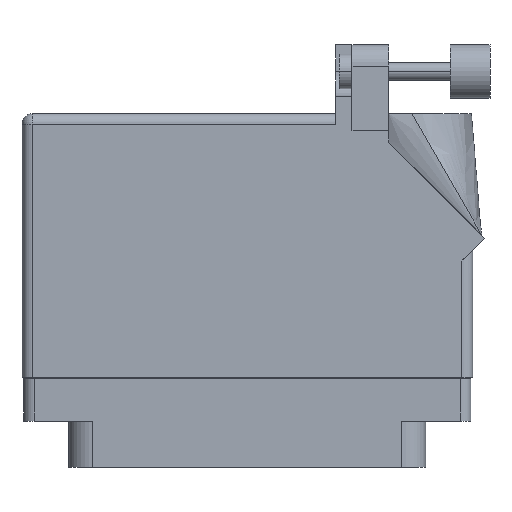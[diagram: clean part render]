
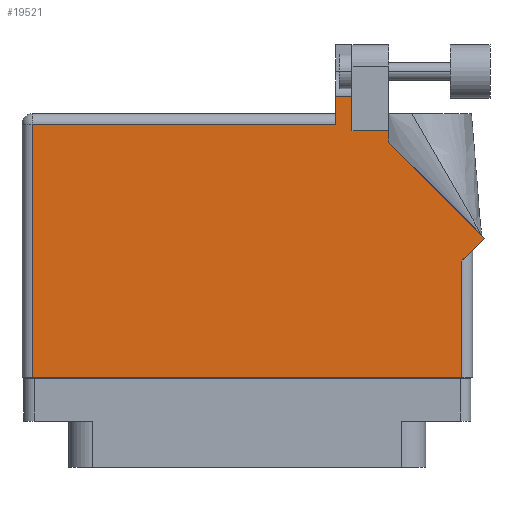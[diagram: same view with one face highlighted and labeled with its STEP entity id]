
A CAD part, front view. The second image highlights one B-rep face of the part: STEP entity #19521.
In plain terms, the highlighted face is planar.
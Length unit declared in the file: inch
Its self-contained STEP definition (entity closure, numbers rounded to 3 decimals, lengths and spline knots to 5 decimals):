
#1962 = DIRECTION ( 'NONE',  ( 0., 1., 0. ) ) ;
#2339 = EDGE_CURVE ( 'NONE', #6748, #19665, #34477, .T. ) ;
#2669 = CARTESIAN_POINT ( 'NONE',  ( -1.306, 1.43, 0.455 ) ) ;
#3012 = PLANE ( 'NONE',  #7684 ) ;
#3174 = ORIENTED_EDGE ( 'NONE', *, *, #38565, .T. ) ;
#3584 = VECTOR ( 'NONE', #25894, 39.37008 ) ;
#3773 = EDGE_CURVE ( 'NONE', #25743, #36689, #9255, .T. ) ;
#3929 = LINE ( 'NONE', #26115, #22565 ) ;
#4601 = CARTESIAN_POINT ( 'NONE',  ( 1.306, 0.637, 0.455 ) ) ;
#5706 = VERTEX_POINT ( 'NONE', #46223 ) ;
#6131 = VECTOR ( 'NONE', #9274, 39.37008 ) ;
#6232 = VECTOR ( 'NONE', #1962, 39.37008 ) ;
#6748 = VERTEX_POINT ( 'NONE', #35886 ) ;
#7314 = ORIENTED_EDGE ( 'NONE', *, *, #37489, .T. ) ;
#7577 = EDGE_LOOP ( 'NONE', ( #7810, #12627, #3174, #16935, #26036, #46610, #27116, #7314, #31782, #34370, #25697 ) ) ;
#7684 = AXIS2_PLACEMENT_3D ( 'NONE', #2669, #29329, #25422 ) ;
#7810 = ORIENTED_EDGE ( 'NONE', *, *, #2339, .T. ) ;
#8013 = DIRECTION ( 'NONE',  ( 1., 0., 0. ) ) ;
#8032 = CARTESIAN_POINT ( 'NONE',  ( 1.244, -0.1, 0.455 ) ) ;
#8064 = VECTOR ( 'NONE', #38087, 39.37008 ) ;
#8741 = VECTOR ( 'NONE', #31526, 39.37008 ) ;
#8875 = VERTEX_POINT ( 'NONE', #41855 ) ;
#9255 = LINE ( 'NONE', #45515, #46002 ) ;
#9274 = DIRECTION ( 'NONE',  ( 0., -1., 0. ) ) ;
#9594 = LINE ( 'NONE', #24406, #6131 ) ;
#9969 = CARTESIAN_POINT ( 'NONE',  ( 1.37671, 0.70771, 0.455 ) ) ;
#12627 = ORIENTED_EDGE ( 'NONE', *, *, #42605, .T. ) ;
#14655 = CARTESIAN_POINT ( 'NONE',  ( 0.93777, 1.5315, 0.455 ) ) ;
#16114 = DIRECTION ( 'NONE',  ( 0.707, 0.707, 0. ) ) ;
#16935 = ORIENTED_EDGE ( 'NONE', *, *, #20073, .T. ) ;
#17822 = EDGE_CURVE ( 'NONE', #8875, #25743, #9594, .T. ) ;
#17823 = VECTOR ( 'NONE', #35160, 39.37008 ) ;
#18857 = CARTESIAN_POINT ( 'NONE',  ( 0.607, 1.33, 0.455 ) ) ;
#19242 = VERTEX_POINT ( 'NONE', #34179 ) ;
#19521 = ADVANCED_FACE ( 'NONE', ( #28025 ), #3012, .F. ) ;
#19665 = VERTEX_POINT ( 'NONE', #40789 ) ;
#20073 = EDGE_CURVE ( 'NONE', #5706, #8875, #26042, .T. ) ;
#20743 = CARTESIAN_POINT ( 'NONE',  ( 0.513, 1.43, 0.455 ) ) ;
#20797 = EDGE_CURVE ( 'NONE', #36689, #28639, #38852, .T. ) ;
#22565 = VECTOR ( 'NONE', #33324, 39.37008 ) ;
#23106 = LINE ( 'NONE', #4601, #41181 ) ;
#23268 = CARTESIAN_POINT ( 'NONE',  ( -1.306, 1.368, 0.455 ) ) ;
#24132 = VERTEX_POINT ( 'NONE', #33546 ) ;
#24406 = CARTESIAN_POINT ( 'NONE',  ( -1.244, -0.1, 0.455 ) ) ;
#24574 = CARTESIAN_POINT ( 'NONE',  ( 1.244, 0.637, 0.455 ) ) ;
#24589 = CARTESIAN_POINT ( 'NONE',  ( 0.82, 1.33, 0.455 ) ) ;
#25422 = DIRECTION ( 'NONE',  ( -1., 0., 0. ) ) ;
#25697 = ORIENTED_EDGE ( 'NONE', *, *, #32283, .T. ) ;
#25743 = VERTEX_POINT ( 'NONE', #42292 ) ;
#25832 = DIRECTION ( 'NONE',  ( 0., 1., 0. ) ) ;
#25894 = DIRECTION ( 'NONE',  ( -1., 0., 0. ) ) ;
#26036 = ORIENTED_EDGE ( 'NONE', *, *, #17822, .T. ) ;
#26042 = LINE ( 'NONE', #23268, #8064 ) ;
#26115 = CARTESIAN_POINT ( 'NONE',  ( 0.82, 1.33, 0.455 ) ) ;
#27116 = ORIENTED_EDGE ( 'NONE', *, *, #20797, .T. ) ;
#27328 = VERTEX_POINT ( 'NONE', #46500 ) ;
#28025 = FACE_OUTER_BOUND ( 'NONE', #7577, .T. ) ;
#28639 = VERTEX_POINT ( 'NONE', #45467 ) ;
#29329 = DIRECTION ( 'NONE',  ( 0., 0., -1. ) ) ;
#29850 = VERTEX_POINT ( 'NONE', #24589 ) ;
#31526 = DIRECTION ( 'NONE',  ( 0., -1., 0. ) ) ;
#31782 = ORIENTED_EDGE ( 'NONE', *, *, #35930, .T. ) ;
#32128 = VECTOR ( 'NONE', #25832, 39.37008 ) ;
#32283 = EDGE_CURVE ( 'NONE', #29850, #6748, #3929, .T. ) ;
#32294 = DIRECTION ( 'NONE',  ( -0.707, 0.707, 0. ) ) ;
#32341 = LINE ( 'NONE', #20743, #8741 ) ;
#33324 = DIRECTION ( 'NONE',  ( -1., 0., 0. ) ) ;
#33546 = CARTESIAN_POINT ( 'NONE',  ( 1.37671, 0.70771, 0.455 ) ) ;
#34070 = EDGE_CURVE ( 'NONE', #19242, #29850, #44072, .T. ) ;
#34179 = CARTESIAN_POINT ( 'NONE',  ( 0.82, 1.26442, 0.455 ) ) ;
#34370 = ORIENTED_EDGE ( 'NONE', *, *, #34070, .T. ) ;
#34477 = LINE ( 'NONE', #18857, #32128 ) ;
#35160 = DIRECTION ( 'NONE',  ( 0., 1., 0. ) ) ;
#35848 = VECTOR ( 'NONE', #32294, 39.37008 ) ;
#35886 = CARTESIAN_POINT ( 'NONE',  ( 0.607, 1.33, 0.455 ) ) ;
#35930 = EDGE_CURVE ( 'NONE', #24132, #19242, #39918, .T. ) ;
#36689 = VERTEX_POINT ( 'NONE', #8032 ) ;
#36805 = LINE ( 'NONE', #14655, #3584 ) ;
#37489 = EDGE_CURVE ( 'NONE', #28639, #24132, #23106, .T. ) ;
#38087 = DIRECTION ( 'NONE',  ( -1., 0., 0. ) ) ;
#38565 = EDGE_CURVE ( 'NONE', #27328, #5706, #32341, .T. ) ;
#38852 = LINE ( 'NONE', #24574, #6232 ) ;
#39918 = LINE ( 'NONE', #9969, #35848 ) ;
#40789 = CARTESIAN_POINT ( 'NONE',  ( 0.607, 1.5315, 0.455 ) ) ;
#41181 = VECTOR ( 'NONE', #16114, 39.37008 ) ;
#41855 = CARTESIAN_POINT ( 'NONE',  ( -1.244, 1.368, 0.455 ) ) ;
#42292 = CARTESIAN_POINT ( 'NONE',  ( -1.244, -0.1, 0.455 ) ) ;
#42605 = EDGE_CURVE ( 'NONE', #19665, #27328, #36805, .T. ) ;
#44072 = LINE ( 'NONE', #44620, #17823 ) ;
#44620 = CARTESIAN_POINT ( 'NONE',  ( 0.82, 1.26442, 0.455 ) ) ;
#45467 = CARTESIAN_POINT ( 'NONE',  ( 1.244, 0.575, 0.455 ) ) ;
#45515 = CARTESIAN_POINT ( 'NONE',  ( -1.306, -0.1, 0.455 ) ) ;
#46002 = VECTOR ( 'NONE', #8013, 39.37008 ) ;
#46223 = CARTESIAN_POINT ( 'NONE',  ( 0.513, 1.368, 0.455 ) ) ;
#46500 = CARTESIAN_POINT ( 'NONE',  ( 0.513, 1.5315, 0.455 ) ) ;
#46610 = ORIENTED_EDGE ( 'NONE', *, *, #3773, .T. ) ;
